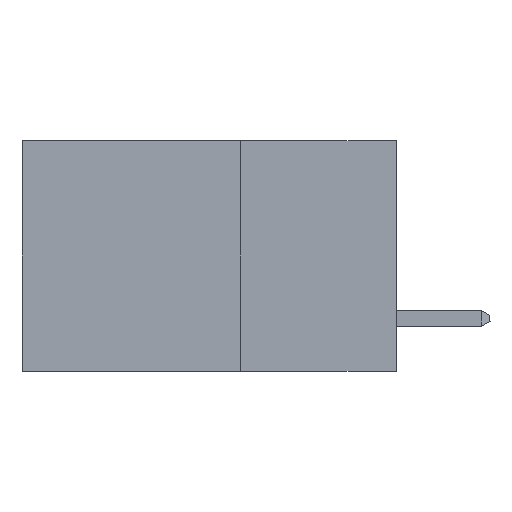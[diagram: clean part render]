
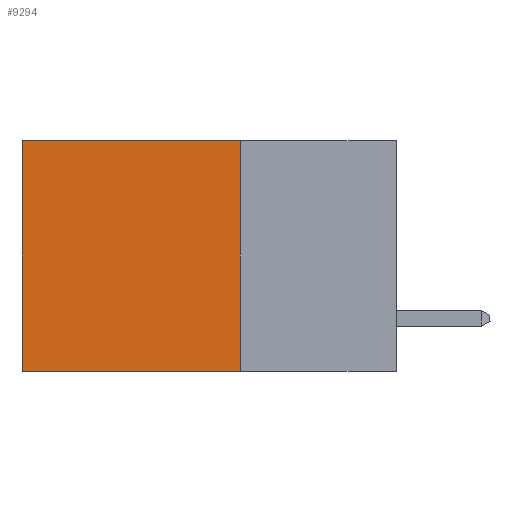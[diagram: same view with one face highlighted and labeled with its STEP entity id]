
A CAD part, left-side view. The second image highlights one B-rep face of the part: STEP entity #9294.
In plain terms, the highlighted planar face has unit normal (-1, 0, 0).
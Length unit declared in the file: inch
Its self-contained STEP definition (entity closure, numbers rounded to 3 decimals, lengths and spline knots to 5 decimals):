
#420 = DIRECTION ( 'NONE',  ( 0., 1., 0. ) ) ;
#979 = EDGE_LOOP ( 'NONE', ( #13672, #27368, #27317, #2632 ) ) ;
#2156 = LINE ( 'NONE', #13637, #3789 ) ;
#2292 = VECTOR ( 'NONE', #420, 39.37008 ) ;
#2632 = ORIENTED_EDGE ( 'NONE', *, *, #25882, .T. ) ;
#3789 = VECTOR ( 'NONE', #11642, 39.37008 ) ;
#4804 = VECTOR ( 'NONE', #27157, 39.37008 ) ;
#5017 = VERTEX_POINT ( 'NONE', #26755 ) ;
#7716 = PLANE ( 'NONE',  #21100 ) ;
#7971 = VERTEX_POINT ( 'NONE', #10476 ) ;
#9029 = CARTESIAN_POINT ( 'NONE',  ( 0.298, 0.25, 0. ) ) ;
#9294 = ADVANCED_FACE ( 'NONE', ( #27574 ), #7716, .F. ) ;
#9831 = CARTESIAN_POINT ( 'NONE',  ( 0.298, 0.25, 0. ) ) ;
#10476 = CARTESIAN_POINT ( 'NONE',  ( 0.298, 0.25, -0.37 ) ) ;
#10843 = CARTESIAN_POINT ( 'NONE',  ( 0.298, 0.25, 0. ) ) ;
#11642 = DIRECTION ( 'NONE',  ( 0., 1., 0. ) ) ;
#12449 = EDGE_CURVE ( 'NONE', #21674, #7971, #27087, .T. ) ;
#13037 = CARTESIAN_POINT ( 'NONE',  ( 0.298, 0.6, 0. ) ) ;
#13637 = CARTESIAN_POINT ( 'NONE',  ( 0.298, 0.25, -0.37 ) ) ;
#13672 = ORIENTED_EDGE ( 'NONE', *, *, #20563, .T. ) ;
#14473 = EDGE_CURVE ( 'NONE', #7971, #5017, #2156, .T. ) ;
#20089 = DIRECTION ( 'NONE',  ( 0., 0., -1. ) ) ;
#20563 = EDGE_CURVE ( 'NONE', #26955, #5017, #23976, .T. ) ;
#20628 = VECTOR ( 'NONE', #21652, 39.37008 ) ;
#21100 = AXIS2_PLACEMENT_3D ( 'NONE', #9831, #26498, #20089 ) ;
#21652 = DIRECTION ( 'NONE',  ( 0., 0., -1. ) ) ;
#21674 = VERTEX_POINT ( 'NONE', #10843 ) ;
#22763 = CARTESIAN_POINT ( 'NONE',  ( 0.298, 0.25, 0. ) ) ;
#23567 = LINE ( 'NONE', #9029, #2292 ) ;
#23608 = CARTESIAN_POINT ( 'NONE',  ( 0.298, 0.6, 0. ) ) ;
#23976 = LINE ( 'NONE', #23608, #20628 ) ;
#25882 = EDGE_CURVE ( 'NONE', #21674, #26955, #23567, .T. ) ;
#26498 = DIRECTION ( 'NONE',  ( 1., 0., 0. ) ) ;
#26755 = CARTESIAN_POINT ( 'NONE',  ( 0.298, 0.6, -0.37 ) ) ;
#26955 = VERTEX_POINT ( 'NONE', #13037 ) ;
#27087 = LINE ( 'NONE', #22763, #4804 ) ;
#27157 = DIRECTION ( 'NONE',  ( 0., 0., -1. ) ) ;
#27317 = ORIENTED_EDGE ( 'NONE', *, *, #12449, .F. ) ;
#27368 = ORIENTED_EDGE ( 'NONE', *, *, #14473, .F. ) ;
#27574 = FACE_OUTER_BOUND ( 'NONE', #979, .T. ) ;
